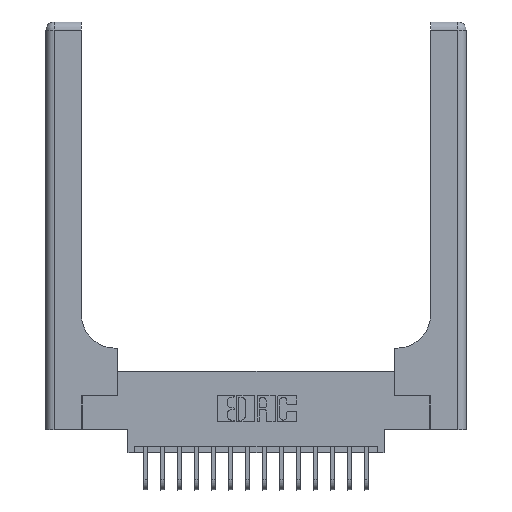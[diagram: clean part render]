
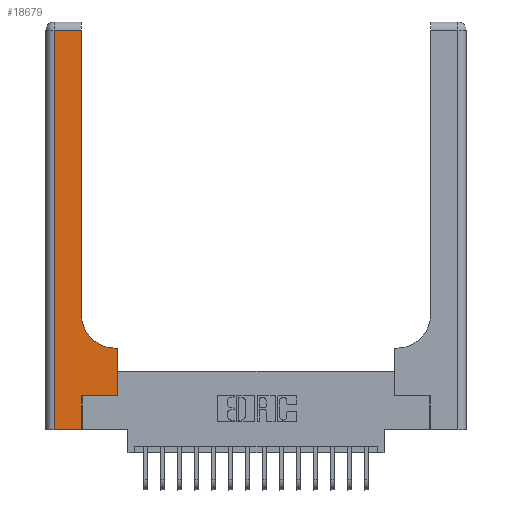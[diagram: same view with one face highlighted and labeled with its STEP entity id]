
A CAD part, top view. The second image highlights one B-rep face of the part: STEP entity #18679.
In plain terms, the highlighted planar face has unit normal (0, 0, 1).
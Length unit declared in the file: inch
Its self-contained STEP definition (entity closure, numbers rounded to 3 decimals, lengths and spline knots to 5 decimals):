
#152 = CARTESIAN_POINT ( 'NONE',  ( 0.51, 0.6, 0.37 ) ) ;
#175 = VERTEX_POINT ( 'NONE', #152 ) ;
#1001 = DIRECTION ( 'NONE',  ( 0., 0., -1. ) ) ;
#1114 = DIRECTION ( 'NONE',  ( -1., 0., 0. ) ) ;
#1275 = EDGE_CURVE ( 'NONE', #5790, #6020, #17145, .T. ) ;
#1329 = EDGE_CURVE ( 'NONE', #7724, #5790, #12209, .T. ) ;
#1358 = EDGE_CURVE ( 'NONE', #13774, #175, #18499, .T. ) ;
#1514 = CARTESIAN_POINT ( 'NONE',  ( 0.51, 0.85, 0.37 ) ) ;
#1527 = EDGE_CURVE ( 'NONE', #3008, #13774, #10119, .T. ) ;
#1668 = VERTEX_POINT ( 'NONE', #2631 ) ;
#1959 = EDGE_CURVE ( 'NONE', #6020, #10854, #15055, .T. ) ;
#2596 = CARTESIAN_POINT ( 'NONE',  ( 0.265, 0.25, 0.37 ) ) ;
#2631 = CARTESIAN_POINT ( 'NONE',  ( 0.26, 0.85, 0.37 ) ) ;
#2657 = CARTESIAN_POINT ( 'NONE',  ( 0.26, 0.6, 0.37 ) ) ;
#2958 = VECTOR ( 'NONE', #10240, 39.37008 ) ;
#3008 = VERTEX_POINT ( 'NONE', #8606 ) ;
#3204 = CARTESIAN_POINT ( 'NONE',  ( 0.26, 2.94, 0.37 ) ) ;
#3532 = CARTESIAN_POINT ( 'NONE',  ( 0.528, 0.6, 0.37 ) ) ;
#3866 = VERTEX_POINT ( 'NONE', #2596 ) ;
#4108 = CARTESIAN_POINT ( 'NONE',  ( 0., 3., 0.37 ) ) ;
#4321 = DIRECTION ( 'NONE',  ( 0., 0., -1. ) ) ;
#4345 = CARTESIAN_POINT ( 'NONE',  ( 0.265, 0., 0.37 ) ) ;
#4423 = DIRECTION ( 'NONE',  ( -1., 0., 0. ) ) ;
#4682 = CIRCLE ( 'NONE', #6995, 0.25 ) ;
#5062 = CARTESIAN_POINT ( 'NONE',  ( 0.265, 0., 0.37 ) ) ;
#5258 = LINE ( 'NONE', #5062, #2958 ) ;
#5267 = CARTESIAN_POINT ( 'NONE',  ( 0.06, 2.94, 0.37 ) ) ;
#5548 = DIRECTION ( 'NONE',  ( 0., 1., 0. ) ) ;
#5712 = ORIENTED_EDGE ( 'NONE', *, *, #14276, .T. ) ;
#5778 = PLANE ( 'NONE',  #16523 ) ;
#5790 = VERTEX_POINT ( 'NONE', #5267 ) ;
#6020 = VERTEX_POINT ( 'NONE', #11054 ) ;
#6182 = CARTESIAN_POINT ( 'NONE',  ( 0., 2.94, 0.37 ) ) ;
#6349 = VECTOR ( 'NONE', #5548, 39.37008 ) ;
#6851 = ORIENTED_EDGE ( 'NONE', *, *, #1358, .T. ) ;
#6995 = AXIS2_PLACEMENT_3D ( 'NONE', #1514, #4321, #16952 ) ;
#7013 = VECTOR ( 'NONE', #16183, 39.37008 ) ;
#7110 = CARTESIAN_POINT ( 'NONE',  ( 0.528, 0.25, 0.37 ) ) ;
#7501 = ORIENTED_EDGE ( 'NONE', *, *, #9636, .T. ) ;
#7524 = VECTOR ( 'NONE', #17269, 39.37008 ) ;
#7724 = VERTEX_POINT ( 'NONE', #3204 ) ;
#8606 = CARTESIAN_POINT ( 'NONE',  ( 0.528, 0.25, 0.37 ) ) ;
#9636 = EDGE_CURVE ( 'NONE', #175, #1668, #4682, .T. ) ;
#9911 = CARTESIAN_POINT ( 'NONE',  ( 0.26, 3., 0.37 ) ) ;
#9976 = VECTOR ( 'NONE', #1114, 39.37008 ) ;
#10119 = LINE ( 'NONE', #7110, #6349 ) ;
#10240 = DIRECTION ( 'NONE',  ( 0., 1., 0. ) ) ;
#10541 = DIRECTION ( 'NONE',  ( 0., -1., 0. ) ) ;
#10854 = VERTEX_POINT ( 'NONE', #4345 ) ;
#10954 = VECTOR ( 'NONE', #16953, 39.37008 ) ;
#11054 = CARTESIAN_POINT ( 'NONE',  ( 0.06, 0., 0.37 ) ) ;
#11678 = LINE ( 'NONE', #9911, #17454 ) ;
#12209 = LINE ( 'NONE', #6182, #10954 ) ;
#12420 = ORIENTED_EDGE ( 'NONE', *, *, #18532, .T. ) ;
#12879 = EDGE_CURVE ( 'NONE', #1668, #7724, #11678, .T. ) ;
#13401 = CARTESIAN_POINT ( 'NONE',  ( 0., 0., 0.37 ) ) ;
#13774 = VERTEX_POINT ( 'NONE', #3532 ) ;
#13856 = LINE ( 'NONE', #14155, #7524 ) ;
#14155 = CARTESIAN_POINT ( 'NONE',  ( 0.265, 0.25, 0.37 ) ) ;
#14276 = EDGE_CURVE ( 'NONE', #3866, #3008, #13856, .T. ) ;
#14806 = ORIENTED_EDGE ( 'NONE', *, *, #1275, .T. ) ;
#15055 = LINE ( 'NONE', #13401, #7013 ) ;
#15077 = DIRECTION ( 'NONE',  ( 0., 1., 0. ) ) ;
#15485 = ORIENTED_EDGE ( 'NONE', *, *, #1959, .T. ) ;
#16120 = ORIENTED_EDGE ( 'NONE', *, *, #1527, .T. ) ;
#16183 = DIRECTION ( 'NONE',  ( 1., 0., 0. ) ) ;
#16188 = ORIENTED_EDGE ( 'NONE', *, *, #12879, .T. ) ;
#16523 = AXIS2_PLACEMENT_3D ( 'NONE', #4108, #1001, #4423 ) ;
#16799 = ORIENTED_EDGE ( 'NONE', *, *, #1329, .T. ) ;
#16896 = EDGE_LOOP ( 'NONE', ( #16188, #16799, #14806, #15485, #12420, #5712, #16120, #6851, #7501 ) ) ;
#16952 = DIRECTION ( 'NONE',  ( 1., 0., 0. ) ) ;
#16953 = DIRECTION ( 'NONE',  ( -1., 0., 0. ) ) ;
#17145 = LINE ( 'NONE', #18798, #17221 ) ;
#17221 = VECTOR ( 'NONE', #10541, 39.37008 ) ;
#17269 = DIRECTION ( 'NONE',  ( 1., 0., 0. ) ) ;
#17454 = VECTOR ( 'NONE', #15077, 39.37008 ) ;
#18499 = LINE ( 'NONE', #2657, #9976 ) ;
#18532 = EDGE_CURVE ( 'NONE', #10854, #3866, #5258, .T. ) ;
#18601 = FACE_OUTER_BOUND ( 'NONE', #16896, .T. ) ;
#18679 = ADVANCED_FACE ( 'NONE', ( #18601 ), #5778, .F. ) ;
#18798 = CARTESIAN_POINT ( 'NONE',  ( 0.06, 3., 0.37 ) ) ;
